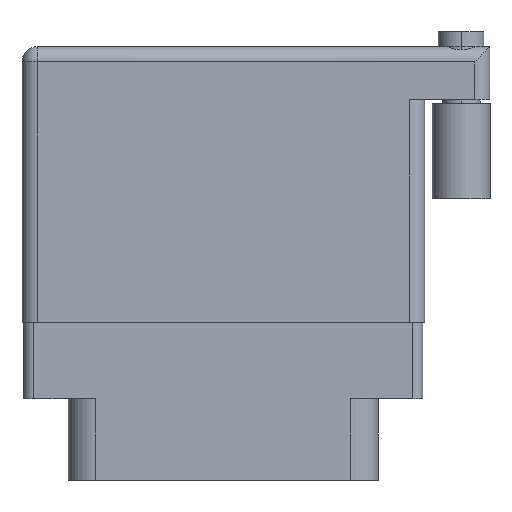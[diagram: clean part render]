
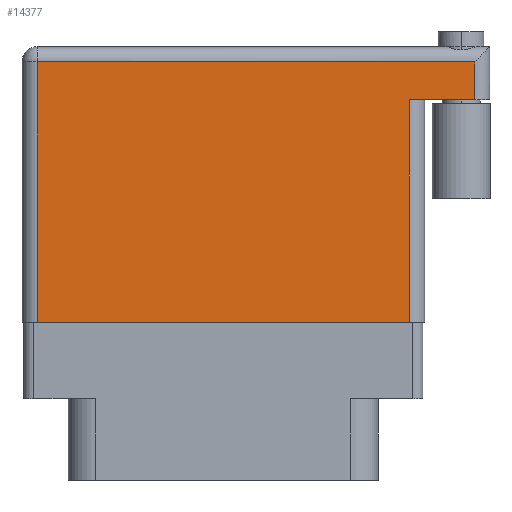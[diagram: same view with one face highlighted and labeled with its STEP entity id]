
A CAD part, front view. The second image highlights one B-rep face of the part: STEP entity #14377.
In plain terms, the highlighted face is planar.
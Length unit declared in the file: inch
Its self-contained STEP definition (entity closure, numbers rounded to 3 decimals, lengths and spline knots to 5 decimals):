
#325 = AXIS2_PLACEMENT_3D ( 'NONE', #6438, #16697, #3652 ) ;
#1242 = ORIENTED_EDGE ( 'NONE', *, *, #1827, .T. ) ;
#1620 = CARTESIAN_POINT ( 'NONE',  ( 1.275, 0.731, 0. ) ) ;
#1827 = EDGE_CURVE ( 'NONE', #3168, #2351, #11826, .T. ) ;
#2351 = VERTEX_POINT ( 'NONE', #4293 ) ;
#2496 = EDGE_LOOP ( 'NONE', ( #5902, #13065, #12903, #1242, #15671, #5965 ) ) ;
#2510 = VERTEX_POINT ( 'NONE', #18829 ) ;
#2552 = FACE_OUTER_BOUND ( 'NONE', #2496, .T. ) ;
#3168 = VERTEX_POINT ( 'NONE', #15133 ) ;
#3652 = DIRECTION ( 'NONE',  ( -1., 0., 0. ) ) ;
#3770 = PLANE ( 'NONE',  #325 ) ;
#4203 = VECTOR ( 'NONE', #14130, 39.37008 ) ;
#4293 = CARTESIAN_POINT ( 'NONE',  ( 1.489, 0.856, 0. ) ) ;
#4587 = VECTOR ( 'NONE', #18159, 39.37008 ) ;
#5414 = CARTESIAN_POINT ( 'NONE',  ( 1.275, 0., 0. ) ) ;
#5902 = ORIENTED_EDGE ( 'NONE', *, *, #6177, .T. ) ;
#5965 = ORIENTED_EDGE ( 'NONE', *, *, #12577, .T. ) ;
#6177 = EDGE_CURVE ( 'NONE', #18020, #11251, #9155, .T. ) ;
#6268 = VECTOR ( 'NONE', #14093, 39.37008 ) ;
#6438 = CARTESIAN_POINT ( 'NONE',  ( 0., 0.906, 0. ) ) ;
#8002 = CARTESIAN_POINT ( 'NONE',  ( 0., 0., 0. ) ) ;
#8094 = LINE ( 'NONE', #17141, #4203 ) ;
#9155 = LINE ( 'NONE', #8002, #4587 ) ;
#10167 = LINE ( 'NONE', #14032, #6268 ) ;
#10444 = VECTOR ( 'NONE', #18323, 39.37008 ) ;
#10919 = CARTESIAN_POINT ( 'NONE',  ( 1.489, 0.906, 0. ) ) ;
#11130 = VECTOR ( 'NONE', #11734, 39.37008 ) ;
#11251 = VERTEX_POINT ( 'NONE', #5414 ) ;
#11734 = DIRECTION ( 'NONE',  ( 0., 1., 0. ) ) ;
#11826 = LINE ( 'NONE', #10919, #10444 ) ;
#11982 = EDGE_CURVE ( 'NONE', #3168, #13626, #10167, .T. ) ;
#12121 = CARTESIAN_POINT ( 'NONE',  ( 1.275, 0.731, 0. ) ) ;
#12205 = LINE ( 'NONE', #17367, #17001 ) ;
#12577 = EDGE_CURVE ( 'NONE', #2510, #18020, #8094, .T. ) ;
#12903 = ORIENTED_EDGE ( 'NONE', *, *, #11982, .F. ) ;
#13065 = ORIENTED_EDGE ( 'NONE', *, *, #16469, .T. ) ;
#13393 = EDGE_CURVE ( 'NONE', #2351, #2510, #12205, .T. ) ;
#13626 = VERTEX_POINT ( 'NONE', #12121 ) ;
#14032 = CARTESIAN_POINT ( 'NONE',  ( 1.539, 0.731, 0. ) ) ;
#14093 = DIRECTION ( 'NONE',  ( -1., 0., 0. ) ) ;
#14130 = DIRECTION ( 'NONE',  ( 0., -1., 0. ) ) ;
#14377 = ADVANCED_FACE ( 'NONE', ( #2552 ), #3770, .F. ) ;
#15020 = LINE ( 'NONE', #1620, #11130 ) ;
#15133 = CARTESIAN_POINT ( 'NONE',  ( 1.489, 0.731, 0. ) ) ;
#15671 = ORIENTED_EDGE ( 'NONE', *, *, #13393, .T. ) ;
#16469 = EDGE_CURVE ( 'NONE', #11251, #13626, #15020, .T. ) ;
#16697 = DIRECTION ( 'NONE',  ( 0., 0., -1. ) ) ;
#17001 = VECTOR ( 'NONE', #18613, 39.37008 ) ;
#17141 = CARTESIAN_POINT ( 'NONE',  ( 0.05, 0., 0. ) ) ;
#17367 = CARTESIAN_POINT ( 'NONE',  ( 0., 0.856, 0. ) ) ;
#18020 = VERTEX_POINT ( 'NONE', #18498 ) ;
#18159 = DIRECTION ( 'NONE',  ( 1., 0., 0. ) ) ;
#18323 = DIRECTION ( 'NONE',  ( 0., 1., 0. ) ) ;
#18498 = CARTESIAN_POINT ( 'NONE',  ( 0.05, 0., 0. ) ) ;
#18613 = DIRECTION ( 'NONE',  ( -1., 0., 0. ) ) ;
#18829 = CARTESIAN_POINT ( 'NONE',  ( 0.05, 0.856, 0. ) ) ;
